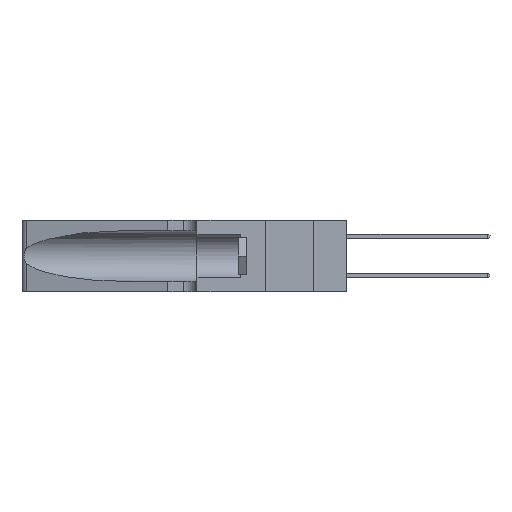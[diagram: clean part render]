
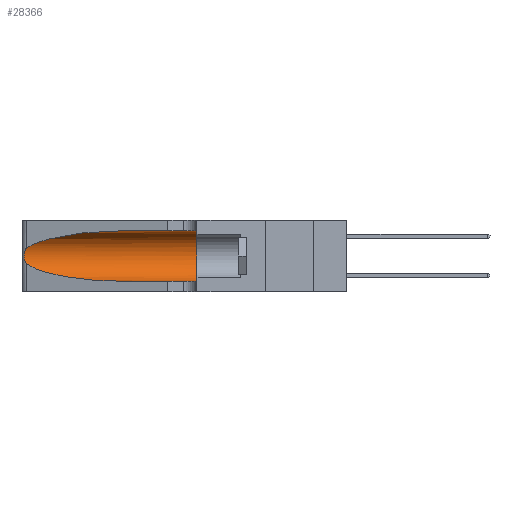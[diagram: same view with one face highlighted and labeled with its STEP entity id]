
A CAD part, left-side view. The second image highlights one B-rep face of the part: STEP entity #28366.
In plain terms, the highlighted cylindrical face has radius 3.308 mm (diameter 6.617 mm), a partial arc.
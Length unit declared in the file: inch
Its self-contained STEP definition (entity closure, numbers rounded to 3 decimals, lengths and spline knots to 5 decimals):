
#77 = DIRECTION ( 'NONE',  ( 0., 1., 0. ) ) ;
#374 = CARTESIAN_POINT ( 'NONE',  ( 0.25856, 1.23593, 0.16098 ) ) ;
#1325 = ORIENTED_EDGE ( 'NONE', *, *, #23687, .T. ) ;
#1585 =( BOUNDED_CURVE ( )  B_SPLINE_CURVE ( 3, ( #14131, #25654, #23394, #16773 ),
 .UNSPECIFIED., .F., .F. ) 
 B_SPLINE_CURVE_WITH_KNOTS ( ( 4, 4 ),
 ( 1.5708, 2.84003 ),
 .UNSPECIFIED. ) 
 CURVE ( )  GEOMETRIC_REPRESENTATION_ITEM ( )  RATIONAL_B_SPLINE_CURVE ( ( 1., 0.87, 0.87, 1. ) ) 
 REPRESENTATION_ITEM ( '' )  );
#1960 = EDGE_CURVE ( 'NONE', #26970, #12561, #19230, .T. ) ;
#2149 = FACE_OUTER_BOUND ( 'NONE', #7652, .T. ) ;
#2247 = VECTOR ( 'NONE', #27538, 39.37008 ) ;
#2638 = EDGE_CURVE ( 'NONE', #8058, #8988, #12583, .T. ) ;
#2849 = CARTESIAN_POINT ( 'NONE',  ( 0.25787, 1.23484, 0.2124 ) ) ;
#4780 = CARTESIAN_POINT ( 'NONE',  ( 0.25487, 1.22718, 0.22369 ) ) ;
#5634 = CARTESIAN_POINT ( 'NONE',  ( 0.1305, 0.72297, 0.05475 ) ) ;
#6823 = CARTESIAN_POINT ( 'NONE',  ( 0.25487, 1.22718, 0.22369 ) ) ;
#7198 = CARTESIAN_POINT ( 'NONE',  ( 0.25639, 1.23186, 0.15144 ) ) ;
#7412 = CARTESIAN_POINT ( 'NONE',  ( 0.25854, 1.2359, 0.20912 ) ) ;
#7526 = CARTESIAN_POINT ( 'NONE',  ( 0.26075, 1.23896, 0.19203 ) ) ;
#7652 = EDGE_LOOP ( 'NONE', ( #15395, #1325, #21831, #28147, #11282, #10755 ) ) ;
#8028 = B_SPLINE_CURVE_WITH_KNOTS ( 'NONE', 3,
 ( #6823, #23910, #21661, #2849, #7412, #23710, #7526, #9789, #9590, #374, #16922, #7198, #26468, #12389 ),
 .UNSPECIFIED., .F., .F.,
 ( 4, 2, 2, 2, 2, 2, 4 ),
 ( 0., 0.00027, 0.00053, 0.00107, 0.0016, 0.00187, 0.00214 ),
 .UNSPECIFIED. ) ;
#8058 = VERTEX_POINT ( 'NONE', #18775 ) ;
#8464 = CARTESIAN_POINT ( 'NONE',  ( 0.1305, 0.35, 0.05475 ) ) ;
#8988 = VERTEX_POINT ( 'NONE', #15938 ) ;
#9590 = CARTESIAN_POINT ( 'NONE',  ( 0.26017, 1.23833, 0.17102 ) ) ;
#9789 = CARTESIAN_POINT ( 'NONE',  ( 0.26075, 1.23896, 0.178 ) ) ;
#10288 = CARTESIAN_POINT ( 'NONE',  ( 0.25487, 1.22718, 0.14631 ) ) ;
#10663 = DIRECTION ( 'NONE',  ( 0., -1., 0. ) ) ;
#10755 = ORIENTED_EDGE ( 'NONE', *, *, #2638, .F. ) ;
#11282 = ORIENTED_EDGE ( 'NONE', *, *, #17908, .F. ) ;
#11336 = DIRECTION ( 'NONE',  ( 0., 0., -1. ) ) ;
#11591 = CARTESIAN_POINT ( 'NONE',  ( 0.1305, 0.72297, 0.05475 ) ) ;
#12389 = CARTESIAN_POINT ( 'NONE',  ( 0.25487, 1.22718, 0.14631 ) ) ;
#12561 = VERTEX_POINT ( 'NONE', #8464 ) ;
#12583 = LINE ( 'NONE', #24970, #13686 ) ;
#13080 = CARTESIAN_POINT ( 'NONE',  ( 0.2373, 1.15595, 0.08982 ) ) ;
#13207 = EDGE_CURVE ( 'NONE', #30088, #26970, #15779, .T. ) ;
#13686 = VECTOR ( 'NONE', #10663, 39.37008 ) ;
#13888 = CARTESIAN_POINT ( 'NONE',  ( 0.1305, 1.61858, 0.185 ) ) ;
#14131 = CARTESIAN_POINT ( 'NONE',  ( 0.1305, 0.72297, 0.31525 ) ) ;
#14414 = AXIS2_PLACEMENT_3D ( 'NONE', #13888, #23060, #11336 ) ;
#15395 = ORIENTED_EDGE ( 'NONE', *, *, #26613, .T. ) ;
#15779 =( BOUNDED_CURVE ( )  B_SPLINE_CURVE ( 3, ( #22441, #13080, #24935, #5634 ),
 .UNSPECIFIED., .F., .F. ) 
 B_SPLINE_CURVE_WITH_KNOTS ( ( 4, 4 ),
 ( 3.44316, 4.71239 ),
 .UNSPECIFIED. ) 
 CURVE ( )  GEOMETRIC_REPRESENTATION_ITEM ( )  RATIONAL_B_SPLINE_CURVE ( ( 1., 0.87, 0.87, 1. ) ) 
 REPRESENTATION_ITEM ( '' )  );
#15938 = CARTESIAN_POINT ( 'NONE',  ( 0.1305, 0.35, 0.31525 ) ) ;
#16611 = VERTEX_POINT ( 'NONE', #4780 ) ;
#16773 = CARTESIAN_POINT ( 'NONE',  ( 0.25487, 1.22718, 0.22369 ) ) ;
#16922 = CARTESIAN_POINT ( 'NONE',  ( 0.25789, 1.23486, 0.15765 ) ) ;
#17308 = CYLINDRICAL_SURFACE ( 'NONE', #14414, 0.13025 ) ;
#17908 = EDGE_CURVE ( 'NONE', #8988, #12561, #27521, .T. ) ;
#18775 = CARTESIAN_POINT ( 'NONE',  ( 0.1305, 0.72297, 0.31525 ) ) ;
#19171 = CARTESIAN_POINT ( 'NONE',  ( 0.1305, 0.35, 0.185 ) ) ;
#19230 = LINE ( 'NONE', #27935, #2247 ) ;
#21133 = DIRECTION ( 'NONE',  ( 0., 0., 1. ) ) ;
#21661 = CARTESIAN_POINT ( 'NONE',  ( 0.25639, 1.23184, 0.21858 ) ) ;
#21831 = ORIENTED_EDGE ( 'NONE', *, *, #13207, .T. ) ;
#22441 = CARTESIAN_POINT ( 'NONE',  ( 0.25487, 1.22718, 0.14631 ) ) ;
#23060 = DIRECTION ( 'NONE',  ( 0., -1., 0. ) ) ;
#23394 = CARTESIAN_POINT ( 'NONE',  ( 0.2373, 1.15595, 0.28018 ) ) ;
#23687 = EDGE_CURVE ( 'NONE', #16611, #30088, #8028, .T. ) ;
#23710 = CARTESIAN_POINT ( 'NONE',  ( 0.26018, 1.23835, 0.19895 ) ) ;
#23910 = CARTESIAN_POINT ( 'NONE',  ( 0.25555, 1.22994, 0.2215 ) ) ;
#24935 = CARTESIAN_POINT ( 'NONE',  ( 0.18966, 0.96281, 0.05475 ) ) ;
#24970 = CARTESIAN_POINT ( 'NONE',  ( 0.1305, 1.61858, 0.31525 ) ) ;
#25654 = CARTESIAN_POINT ( 'NONE',  ( 0.18966, 0.96281, 0.31525 ) ) ;
#26468 = CARTESIAN_POINT ( 'NONE',  ( 0.25555, 1.22993, 0.14849 ) ) ;
#26613 = EDGE_CURVE ( 'NONE', #8058, #16611, #1585, .T. ) ;
#26970 = VERTEX_POINT ( 'NONE', #11591 ) ;
#27521 = CIRCLE ( 'NONE', #28023, 0.13025 ) ;
#27538 = DIRECTION ( 'NONE',  ( 0., -1., 0. ) ) ;
#27935 = CARTESIAN_POINT ( 'NONE',  ( 0.1305, 1.61858, 0.05475 ) ) ;
#28023 = AXIS2_PLACEMENT_3D ( 'NONE', #19171, #77, #21133 ) ;
#28147 = ORIENTED_EDGE ( 'NONE', *, *, #1960, .T. ) ;
#28366 = ADVANCED_FACE ( 'NONE', ( #2149 ), #17308, .F. ) ;
#30088 = VERTEX_POINT ( 'NONE', #10288 ) ;
